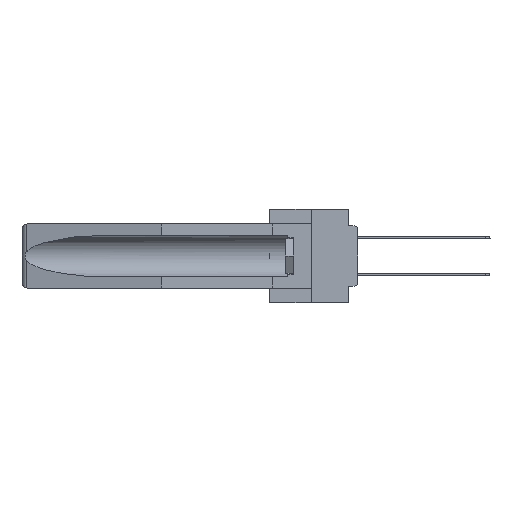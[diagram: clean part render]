
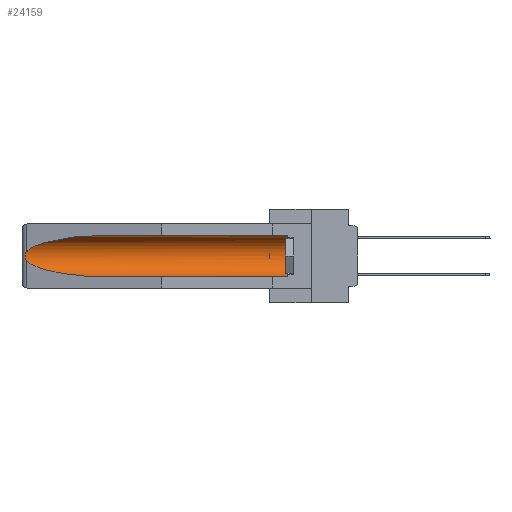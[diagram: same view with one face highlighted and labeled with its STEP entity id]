
A CAD part, left-side view. The second image highlights one B-rep face of the part: STEP entity #24159.
In plain terms, the highlighted cylindrical face has radius 2.857 mm (diameter 5.715 mm), a partial arc.
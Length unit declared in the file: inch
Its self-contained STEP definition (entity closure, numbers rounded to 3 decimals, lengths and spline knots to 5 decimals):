
#1804 = VERTEX_POINT ( 'NONE', #8363 ) ;
#2525 = EDGE_CURVE ( 'NONE', #9808, #19452, #3518, .T. ) ;
#2546 = DIRECTION ( 'NONE',  ( 0., 0., 1. ) ) ;
#2561 = ORIENTED_EDGE ( 'NONE', *, *, #25343, .T. ) ;
#2626 = CARTESIAN_POINT ( 'NONE',  ( 0.25451, 1.48313, -0.24835 ) ) ;
#2854 = CYLINDRICAL_SURFACE ( 'NONE', #25590, 0.1125 ) ;
#3518 = B_SPLINE_CURVE_WITH_KNOTS ( 'NONE', 3,
 ( #31187, #16191, #38471, #9375, #9506, #9758, #35187, #15818, #9629, #38354 ),
 .UNSPECIFIED., .F., .F.,
 ( 4, 2, 2, 2, 4 ),
 ( 0., 0.00029, 0.00058, 0.00087, 0.00117 ),
 .UNSPECIFIED. ) ;
#3935 = EDGE_CURVE ( 'NONE', #34498, #9808, #4808, .T. ) ;
#4262 =( BOUNDED_CURVE ( )  B_SPLINE_CURVE ( 3, ( #21793, #2626, #40677, #28329 ),
 .UNSPECIFIED., .F., .F. ) 
 B_SPLINE_CURVE_WITH_KNOTS ( ( 4, 4 ),
 ( 0.1948, 1.5708 ),
 .UNSPECIFIED. ) 
 CURVE ( )  GEOMETRIC_REPRESENTATION_ITEM ( )  RATIONAL_B_SPLINE_CURVE ( ( 1., 0.848, 0.848, 1. ) ) 
 REPRESENTATION_ITEM ( '' )  );
#4606 = VECTOR ( 'NONE', #7942, 39.37008 ) ;
#4808 =( BOUNDED_CURVE ( )  B_SPLINE_CURVE ( 3, ( #14936, #30446, #17866, #37256 ),
 .UNSPECIFIED., .F., .F. ) 
 B_SPLINE_CURVE_WITH_KNOTS ( ( 4, 4 ),
 ( 4.71239, 6.08839 ),
 .UNSPECIFIED. ) 
 CURVE ( )  GEOMETRIC_REPRESENTATION_ITEM ( )  RATIONAL_B_SPLINE_CURVE ( ( 1., 0.848, 0.848, 1. ) ) 
 REPRESENTATION_ITEM ( '' )  );
#6155 = ORIENTED_EDGE ( 'NONE', *, *, #25378, .T. ) ;
#7942 = DIRECTION ( 'NONE',  ( 0., 1., 0. ) ) ;
#8248 = CARTESIAN_POINT ( 'NONE',  ( 0.26537, 1.52718, -0.19328 ) ) ;
#8363 = CARTESIAN_POINT ( 'NONE',  ( 0.155, 0.126, -0.059 ) ) ;
#9375 = CARTESIAN_POINT ( 'NONE',  ( 0.2673, 1.5327, -0.16383 ) ) ;
#9506 = CARTESIAN_POINT ( 'NONE',  ( 0.2675, 1.53308, -0.16763 ) ) ;
#9629 = CARTESIAN_POINT ( 'NONE',  ( 0.26597, 1.5296, -0.19026 ) ) ;
#9758 = CARTESIAN_POINT ( 'NONE',  ( 0.2675, 1.53308, -0.17534 ) ) ;
#9808 = VERTEX_POINT ( 'NONE', #27481 ) ;
#10794 = FACE_OUTER_BOUND ( 'NONE', #12978, .T. ) ;
#10834 = ORIENTED_EDGE ( 'NONE', *, *, #2525, .T. ) ;
#11488 = AXIS2_PLACEMENT_3D ( 'NONE', #18753, #31181, #2546 ) ;
#12430 = DIRECTION ( 'NONE',  ( 0., 0., 1. ) ) ;
#12460 = LINE ( 'NONE', #31413, #22004 ) ;
#12978 = EDGE_LOOP ( 'NONE', ( #17223, #10834, #2561, #25584, #6155, #32788 ) ) ;
#14502 = CIRCLE ( 'NONE', #11488, 0.1125 ) ;
#14936 = CARTESIAN_POINT ( 'NONE',  ( 0.155, 1.07973, -0.059 ) ) ;
#15497 = DIRECTION ( 'NONE',  ( 0., 1., 0. ) ) ;
#15818 = CARTESIAN_POINT ( 'NONE',  ( 0.26655, 1.53094, -0.18657 ) ) ;
#16191 = CARTESIAN_POINT ( 'NONE',  ( 0.26597, 1.52961, -0.15275 ) ) ;
#17223 = ORIENTED_EDGE ( 'NONE', *, *, #3935, .T. ) ;
#17866 = CARTESIAN_POINT ( 'NONE',  ( 0.25451, 1.48313, -0.09465 ) ) ;
#18753 = CARTESIAN_POINT ( 'NONE',  ( 0.155, 0.126, -0.1715 ) ) ;
#19452 = VERTEX_POINT ( 'NONE', #8248 ) ;
#19538 = EDGE_CURVE ( 'NONE', #19783, #22215, #12460, .T. ) ;
#19783 = VERTEX_POINT ( 'NONE', #39923 ) ;
#20031 = CARTESIAN_POINT ( 'NONE',  ( 0.155, 1.07973, -0.284 ) ) ;
#21793 = CARTESIAN_POINT ( 'NONE',  ( 0.26537, 1.52718, -0.19328 ) ) ;
#22004 = VECTOR ( 'NONE', #15497, 39.37008 ) ;
#22215 = VERTEX_POINT ( 'NONE', #20031 ) ;
#24133 = LINE ( 'NONE', #27129, #4606 ) ;
#24159 = ADVANCED_FACE ( 'NONE', ( #10794 ), #2854, .F. ) ;
#25170 = CARTESIAN_POINT ( 'NONE',  ( 0.155, -0.30754, -0.1715 ) ) ;
#25343 = EDGE_CURVE ( 'NONE', #19452, #22215, #4262, .T. ) ;
#25378 = EDGE_CURVE ( 'NONE', #19783, #1804, #14502, .T. ) ;
#25584 = ORIENTED_EDGE ( 'NONE', *, *, #19538, .F. ) ;
#25590 = AXIS2_PLACEMENT_3D ( 'NONE', #25170, #35174, #12430 ) ;
#26515 = EDGE_CURVE ( 'NONE', #1804, #34498, #24133, .T. ) ;
#27129 = CARTESIAN_POINT ( 'NONE',  ( 0.155, -0.30754, -0.059 ) ) ;
#27287 = CARTESIAN_POINT ( 'NONE',  ( 0.155, 1.07973, -0.059 ) ) ;
#27481 = CARTESIAN_POINT ( 'NONE',  ( 0.26537, 1.52718, -0.14972 ) ) ;
#28329 = CARTESIAN_POINT ( 'NONE',  ( 0.155, 1.07973, -0.284 ) ) ;
#30446 = CARTESIAN_POINT ( 'NONE',  ( 0.21114, 1.30732, -0.059 ) ) ;
#31181 = DIRECTION ( 'NONE',  ( 0., -1., 0. ) ) ;
#31187 = CARTESIAN_POINT ( 'NONE',  ( 0.26537, 1.52718, -0.14972 ) ) ;
#31413 = CARTESIAN_POINT ( 'NONE',  ( 0.155, -0.30754, -0.284 ) ) ;
#32788 = ORIENTED_EDGE ( 'NONE', *, *, #26515, .T. ) ;
#34498 = VERTEX_POINT ( 'NONE', #27287 ) ;
#35174 = DIRECTION ( 'NONE',  ( 0., 1., 0. ) ) ;
#35187 = CARTESIAN_POINT ( 'NONE',  ( 0.2673, 1.53269, -0.17917 ) ) ;
#37256 = CARTESIAN_POINT ( 'NONE',  ( 0.26537, 1.52718, -0.14972 ) ) ;
#38354 = CARTESIAN_POINT ( 'NONE',  ( 0.26537, 1.52718, -0.19328 ) ) ;
#38471 = CARTESIAN_POINT ( 'NONE',  ( 0.26654, 1.53092, -0.15636 ) ) ;
#39923 = CARTESIAN_POINT ( 'NONE',  ( 0.155, 0.126, -0.284 ) ) ;
#40677 = CARTESIAN_POINT ( 'NONE',  ( 0.21114, 1.30732, -0.284 ) ) ;
